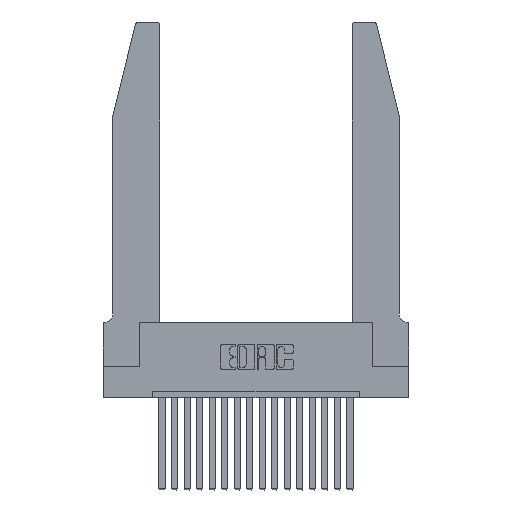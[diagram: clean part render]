
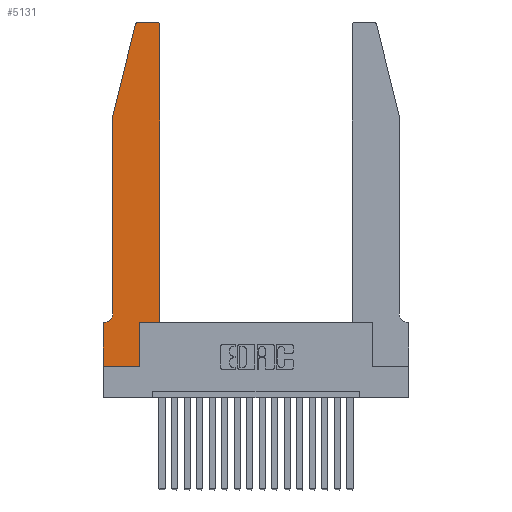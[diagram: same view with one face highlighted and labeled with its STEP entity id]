
A CAD part, top view. The second image highlights one B-rep face of the part: STEP entity #5131.
In plain terms, the highlighted planar face has unit normal (0, 0, 1).
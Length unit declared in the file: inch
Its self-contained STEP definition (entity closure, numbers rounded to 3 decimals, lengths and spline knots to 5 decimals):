
#338 = CARTESIAN_POINT ( 'NONE',  ( 0., 0., 0.37 ) ) ;
#362 = VECTOR ( 'NONE', #8371, 39.37008 ) ;
#509 = DIRECTION ( 'NONE',  ( 0., 0., -1. ) ) ;
#656 = CARTESIAN_POINT ( 'NONE',  ( 0.2605, 2.75, 0.37 ) ) ;
#1623 = EDGE_CURVE ( 'NONE', #8956, #9263, #3269, .T. ) ;
#1642 = ORIENTED_EDGE ( 'NONE', *, *, #3456, .T. ) ;
#1657 = VECTOR ( 'NONE', #16369, 39.37008 ) ;
#1715 = ORIENTED_EDGE ( 'NONE', *, *, #8992, .T. ) ;
#1755 = DIRECTION ( 'NONE',  ( 1., 0., 0. ) ) ;
#1973 = CARTESIAN_POINT ( 'NONE',  ( 0.284, 2.75, 0.37 ) ) ;
#2049 = DIRECTION ( 'NONE',  ( 1., 0., 0. ) ) ;
#2364 = EDGE_CURVE ( 'NONE', #16915, #12674, #16639, .T. ) ;
#2395 = DIRECTION ( 'NONE',  ( 0., -1., 0. ) ) ;
#2453 = CARTESIAN_POINT ( 'NONE',  ( 0., 0.35, 0.37 ) ) ;
#2710 = VECTOR ( 'NONE', #12732, 39.37008 ) ;
#3269 = LINE ( 'NONE', #11326, #14904 ) ;
#3456 = EDGE_CURVE ( 'NONE', #5514, #14393, #3746, .T. ) ;
#3591 = CARTESIAN_POINT ( 'NONE',  ( 0.0055, 0.42, 0.37 ) ) ;
#3746 = LINE ( 'NONE', #14116, #15852 ) ;
#3822 = LINE ( 'NONE', #11703, #17883 ) ;
#4672 = CARTESIAN_POINT ( 'NONE',  ( 0.4505, 2.72, 0.37 ) ) ;
#5027 = AXIS2_PLACEMENT_3D ( 'NONE', #3591, #509, #5232 ) ;
#5131 = ADVANCED_FACE ( 'NONE', ( #8015 ), #15024, .T. ) ;
#5232 = DIRECTION ( 'NONE',  ( -1., 0., 0. ) ) ;
#5307 = DIRECTION ( 'NONE',  ( -1., 0., 0. ) ) ;
#5452 = LINE ( 'NONE', #15661, #14380 ) ;
#5495 = ORIENTED_EDGE ( 'NONE', *, *, #11832, .T. ) ;
#5514 = VERTEX_POINT ( 'NONE', #11502 ) ;
#5979 = DIRECTION ( 'NONE',  ( 1., 0., 0. ) ) ;
#6049 = EDGE_CURVE ( 'NONE', #18287, #6109, #18419, .T. ) ;
#6051 = LINE ( 'NONE', #16319, #12096 ) ;
#6109 = VERTEX_POINT ( 'NONE', #2453 ) ;
#6510 = CARTESIAN_POINT ( 'NONE',  ( 0.0755, 2., 0.37 ) ) ;
#6974 = CARTESIAN_POINT ( 'NONE',  ( 0.0755, 0.42, 0.37 ) ) ;
#7217 = VERTEX_POINT ( 'NONE', #8789 ) ;
#7219 = CARTESIAN_POINT ( 'NONE',  ( 0.2865, 0.35, 0.37 ) ) ;
#8015 = FACE_OUTER_BOUND ( 'NONE', #12821, .T. ) ;
#8044 = DIRECTION ( 'NONE',  ( 0., 1., 0. ) ) ;
#8308 = DIRECTION ( 'NONE',  ( 0., 0., 1. ) ) ;
#8312 = AXIS2_PLACEMENT_3D ( 'NONE', #17682, #8308, #2049 ) ;
#8371 = DIRECTION ( 'NONE',  ( 0., 1., 0. ) ) ;
#8388 = DIRECTION ( 'NONE',  ( 1., 0., 0. ) ) ;
#8789 = CARTESIAN_POINT ( 'NONE',  ( 0.4505, 0.35, 0.37 ) ) ;
#8956 = VERTEX_POINT ( 'NONE', #17018 ) ;
#8992 = EDGE_CURVE ( 'NONE', #13745, #16915, #15503, .T. ) ;
#9242 = VERTEX_POINT ( 'NONE', #338 ) ;
#9250 = CARTESIAN_POINT ( 'NONE',  ( 0.0055, 0.35, 0.37 ) ) ;
#9263 = VERTEX_POINT ( 'NONE', #6974 ) ;
#9278 = CARTESIAN_POINT ( 'NONE',  ( 0.4205, 2.75, 0.37 ) ) ;
#9287 = ORIENTED_EDGE ( 'NONE', *, *, #6049, .T. ) ;
#9354 = ORIENTED_EDGE ( 'NONE', *, *, #1623, .T. ) ;
#9444 = ORIENTED_EDGE ( 'NONE', *, *, #17898, .T. ) ;
#9642 = ORIENTED_EDGE ( 'NONE', *, *, #18826, .T. ) ;
#9779 = VERTEX_POINT ( 'NONE', #4672 ) ;
#10252 = EDGE_CURVE ( 'NONE', #9242, #5514, #6051, .T. ) ;
#10375 = DIRECTION ( 'NONE',  ( 1., 0., 0. ) ) ;
#10412 = CARTESIAN_POINT ( 'NONE',  ( 0.0755, 0.35, 0.37 ) ) ;
#10590 = CIRCLE ( 'NONE', #10716, 0.03 ) ;
#10716 = AXIS2_PLACEMENT_3D ( 'NONE', #19684, #13527, #10375 ) ;
#10755 = CIRCLE ( 'NONE', #5027, 0.07 ) ;
#11236 = LINE ( 'NONE', #6510, #2710 ) ;
#11326 = CARTESIAN_POINT ( 'NONE',  ( 0.0755, 2., 0.37 ) ) ;
#11462 = DIRECTION ( 'NONE',  ( 0., -1., 0. ) ) ;
#11502 = CARTESIAN_POINT ( 'NONE',  ( 0.2865, 0., 0.37 ) ) ;
#11531 = LINE ( 'NONE', #19321, #362 ) ;
#11703 = CARTESIAN_POINT ( 'NONE',  ( 0., 0., 0.37 ) ) ;
#11832 = EDGE_CURVE ( 'NONE', #9779, #13745, #10590, .T. ) ;
#12096 = VECTOR ( 'NONE', #8388, 39.37008 ) ;
#12674 = VERTEX_POINT ( 'NONE', #15450 ) ;
#12732 = DIRECTION ( 'NONE',  ( -0.239, -0.971, 0. ) ) ;
#12770 = ORIENTED_EDGE ( 'NONE', *, *, #13867, .T. ) ;
#12821 = EDGE_LOOP ( 'NONE', ( #1715, #17854, #12770, #9354, #13605, #9287, #16601, #16282, #1642, #9642, #9444, #5495 ) ) ;
#13527 = DIRECTION ( 'NONE',  ( 0., 0., 1. ) ) ;
#13605 = ORIENTED_EDGE ( 'NONE', *, *, #13896, .T. ) ;
#13745 = VERTEX_POINT ( 'NONE', #9278 ) ;
#13867 = EDGE_CURVE ( 'NONE', #12674, #8956, #11236, .T. ) ;
#13896 = EDGE_CURVE ( 'NONE', #9263, #18287, #10755, .T. ) ;
#14116 = CARTESIAN_POINT ( 'NONE',  ( 0.2865, 0.35, 0.37 ) ) ;
#14380 = VECTOR ( 'NONE', #1755, 39.37008 ) ;
#14393 = VERTEX_POINT ( 'NONE', #7219 ) ;
#14904 = VECTOR ( 'NONE', #11462, 39.37008 ) ;
#15024 = PLANE ( 'NONE',  #18645 ) ;
#15094 = CARTESIAN_POINT ( 'NONE',  ( 0., 0.35, 0.37 ) ) ;
#15450 = CARTESIAN_POINT ( 'NONE',  ( 0.25487, 2.72718, 0.37 ) ) ;
#15503 = LINE ( 'NONE', #656, #16538 ) ;
#15661 = CARTESIAN_POINT ( 'NONE',  ( 0.4505, 0.35, 0.37 ) ) ;
#15852 = VECTOR ( 'NONE', #8044, 39.37008 ) ;
#16282 = ORIENTED_EDGE ( 'NONE', *, *, #10252, .T. ) ;
#16319 = CARTESIAN_POINT ( 'NONE',  ( 0., 0., 0.37 ) ) ;
#16369 = DIRECTION ( 'NONE',  ( -1., 0., 0. ) ) ;
#16538 = VECTOR ( 'NONE', #5307, 39.37008 ) ;
#16601 = ORIENTED_EDGE ( 'NONE', *, *, #17246, .T. ) ;
#16639 = CIRCLE ( 'NONE', #8312, 0.03 ) ;
#16915 = VERTEX_POINT ( 'NONE', #1973 ) ;
#17018 = CARTESIAN_POINT ( 'NONE',  ( 0.0755, 2., 0.37 ) ) ;
#17246 = EDGE_CURVE ( 'NONE', #6109, #9242, #3822, .T. ) ;
#17682 = CARTESIAN_POINT ( 'NONE',  ( 0.284, 2.72, 0.37 ) ) ;
#17854 = ORIENTED_EDGE ( 'NONE', *, *, #2364, .T. ) ;
#17883 = VECTOR ( 'NONE', #2395, 39.37008 ) ;
#17898 = EDGE_CURVE ( 'NONE', #7217, #9779, #11531, .T. ) ;
#18287 = VERTEX_POINT ( 'NONE', #9250 ) ;
#18419 = LINE ( 'NONE', #10412, #1657 ) ;
#18445 = DIRECTION ( 'NONE',  ( 0., 0., 1. ) ) ;
#18645 = AXIS2_PLACEMENT_3D ( 'NONE', #15094, #18445, #5979 ) ;
#18826 = EDGE_CURVE ( 'NONE', #14393, #7217, #5452, .T. ) ;
#19321 = CARTESIAN_POINT ( 'NONE',  ( 0.4505, 0.35, 0.37 ) ) ;
#19684 = CARTESIAN_POINT ( 'NONE',  ( 0.4205, 2.72, 0.37 ) ) ;
